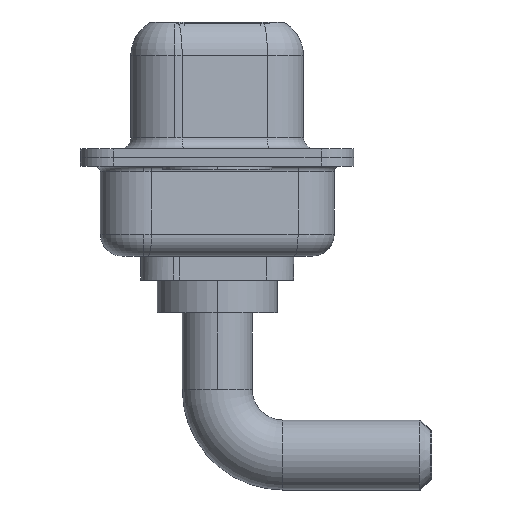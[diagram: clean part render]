
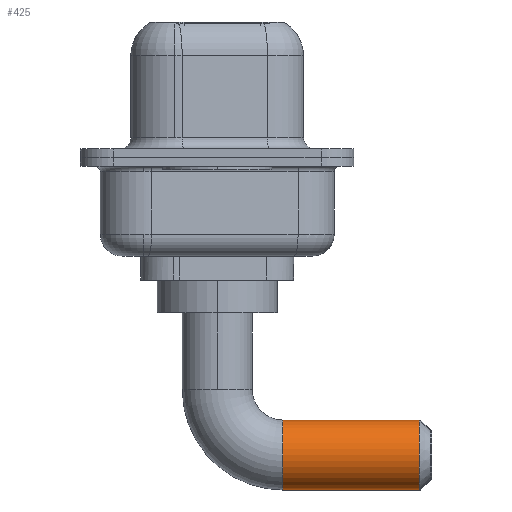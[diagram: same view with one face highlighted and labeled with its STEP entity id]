
A CAD part, left-side view. The second image highlights one B-rep face of the part: STEP entity #425.
In plain terms, the highlighted cylindrical face has radius 1.6 mm (diameter 3.2 mm), a partial arc.
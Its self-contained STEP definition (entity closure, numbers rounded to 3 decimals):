
#295 = CYLINDRICAL_SURFACE ( 'NONE', #1244, 1.6 ) ;
#425 = ADVANCED_FACE ( 'NONE', ( #2820 ), #295, .T. ) ;
#481 = DIRECTION ( 'NONE',  ( -1., 0., 0. ) ) ;
#769 = EDGE_CURVE ( 'NONE', #3917, #9408, #6054, .T. ) ;
#1244 = AXIS2_PLACEMENT_3D ( 'NONE', #10035, #7342, #6413 ) ;
#1424 = CIRCLE ( 'NONE', #7938, 1.6 ) ;
#2283 = ORIENTED_EDGE ( 'NONE', *, *, #10180, .F. ) ;
#2546 = VERTEX_POINT ( 'NONE', #9488 ) ;
#2638 = VECTOR ( 'NONE', #6155, 1000. ) ;
#2820 = FACE_OUTER_BOUND ( 'NONE', #7118, .T. ) ;
#2870 = CARTESIAN_POINT ( 'NONE',  ( 0., -9.25, -8.1 ) ) ;
#3134 = VECTOR ( 'NONE', #5251, 1000. ) ;
#3181 = CIRCLE ( 'NONE', #9674, 1.6 ) ;
#3458 = ORIENTED_EDGE ( 'NONE', *, *, #4204, .T. ) ;
#3917 = VERTEX_POINT ( 'NONE', #4547 ) ;
#4109 = CARTESIAN_POINT ( 'NONE',  ( 0., -9.25, -6.5 ) ) ;
#4169 = ORIENTED_EDGE ( 'NONE', *, *, #5589, .T. ) ;
#4204 = EDGE_CURVE ( 'NONE', #9408, #2546, #3181, .T. ) ;
#4267 = CARTESIAN_POINT ( 'NONE',  ( 0., -3., -8.1 ) ) ;
#4547 = CARTESIAN_POINT ( 'NONE',  ( 0., -3., -8.1 ) ) ;
#4887 = ORIENTED_EDGE ( 'NONE', *, *, #769, .T. ) ;
#5251 = DIRECTION ( 'NONE',  ( 0., -1., 0. ) ) ;
#5589 = EDGE_CURVE ( 'NONE', #5606, #3917, #1424, .T. ) ;
#5606 = VERTEX_POINT ( 'NONE', #7769 ) ;
#6054 = LINE ( 'NONE', #4267, #3134 ) ;
#6155 = DIRECTION ( 'NONE',  ( 0., -1., 0. ) ) ;
#6413 = DIRECTION ( 'NONE',  ( 0., 0., -1. ) ) ;
#7118 = EDGE_LOOP ( 'NONE', ( #2283, #4169, #4887, #3458 ) ) ;
#7342 = DIRECTION ( 'NONE',  ( 0., -1., 0. ) ) ;
#7652 = DIRECTION ( 'NONE',  ( 0., 0., -1. ) ) ;
#7764 = DIRECTION ( 'NONE',  ( 0., 1., 0. ) ) ;
#7769 = CARTESIAN_POINT ( 'NONE',  ( 0., -3., -4.9 ) ) ;
#7938 = AXIS2_PLACEMENT_3D ( 'NONE', #11152, #8594, #481 ) ;
#8594 = DIRECTION ( 'NONE',  ( 0., -1., 0. ) ) ;
#9408 = VERTEX_POINT ( 'NONE', #2870 ) ;
#9488 = CARTESIAN_POINT ( 'NONE',  ( 0., -9.25, -4.9 ) ) ;
#9589 = LINE ( 'NONE', #9651, #2638 ) ;
#9651 = CARTESIAN_POINT ( 'NONE',  ( 0., -3., -4.9 ) ) ;
#9674 = AXIS2_PLACEMENT_3D ( 'NONE', #4109, #7764, #7652 ) ;
#10035 = CARTESIAN_POINT ( 'NONE',  ( 0., -3., -6.5 ) ) ;
#10180 = EDGE_CURVE ( 'NONE', #5606, #2546, #9589, .T. ) ;
#11152 = CARTESIAN_POINT ( 'NONE',  ( 0., -3., -6.5 ) ) ;
